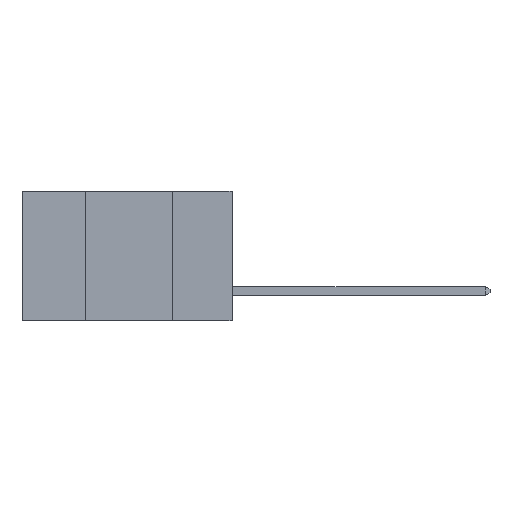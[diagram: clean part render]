
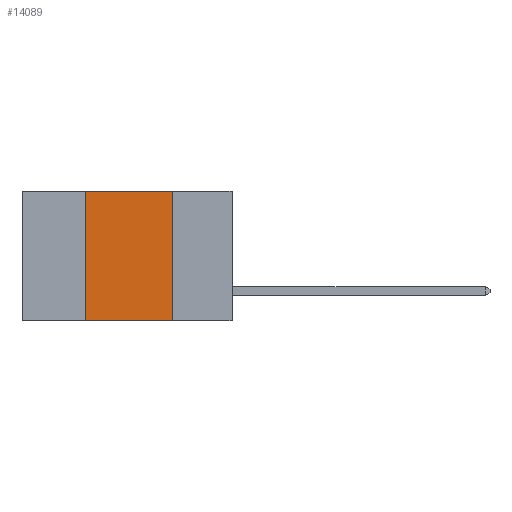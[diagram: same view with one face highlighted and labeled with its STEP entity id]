
A CAD part, left-side view. The second image highlights one B-rep face of the part: STEP entity #14089.
In plain terms, the highlighted planar face has unit normal (-1, 0, 0).
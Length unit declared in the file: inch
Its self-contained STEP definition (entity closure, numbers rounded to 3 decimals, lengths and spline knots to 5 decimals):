
#72 = EDGE_LOOP ( 'NONE', ( #18517, #10150, #10084, #10769 ) ) ;
#1150 = EDGE_CURVE ( 'NONE', #11482, #13992, #9369, .T. ) ;
#1518 = VECTOR ( 'NONE', #13849, 39.37008 ) ;
#2031 = LINE ( 'NONE', #8799, #1518 ) ;
#2563 = AXIS2_PLACEMENT_3D ( 'NONE', #2743, #13719, #4466 ) ;
#2743 = CARTESIAN_POINT ( 'NONE',  ( 0., 0.6, 0. ) ) ;
#3297 = LINE ( 'NONE', #7879, #18875 ) ;
#3384 = EDGE_CURVE ( 'NONE', #13992, #12491, #2031, .T. ) ;
#4466 = DIRECTION ( 'NONE',  ( 0., 0., -1. ) ) ;
#4492 = EDGE_CURVE ( 'NONE', #11482, #5430, #3297, .T. ) ;
#5430 = VERTEX_POINT ( 'NONE', #15774 ) ;
#6145 = VECTOR ( 'NONE', #15938, 39.37008 ) ;
#6451 = LINE ( 'NONE', #11126, #14081 ) ;
#6978 = FACE_OUTER_BOUND ( 'NONE', #72, .T. ) ;
#7617 = PLANE ( 'NONE',  #2563 ) ;
#7879 = CARTESIAN_POINT ( 'NONE',  ( 0., 0.6, -0.37 ) ) ;
#8799 = CARTESIAN_POINT ( 'NONE',  ( 0., 0.6, 0. ) ) ;
#9068 = DIRECTION ( 'NONE',  ( 0., -1., 0. ) ) ;
#9369 = LINE ( 'NONE', #15669, #6145 ) ;
#9662 = DIRECTION ( 'NONE',  ( 0., 0., -1. ) ) ;
#10084 = ORIENTED_EDGE ( 'NONE', *, *, #1150, .F. ) ;
#10150 = ORIENTED_EDGE ( 'NONE', *, *, #3384, .F. ) ;
#10769 = ORIENTED_EDGE ( 'NONE', *, *, #4492, .T. ) ;
#11126 = CARTESIAN_POINT ( 'NONE',  ( 0., 0.17, 0. ) ) ;
#11482 = VERTEX_POINT ( 'NONE', #14556 ) ;
#12491 = VERTEX_POINT ( 'NONE', #18179 ) ;
#13467 = CARTESIAN_POINT ( 'NONE',  ( 0., 0.42, 0. ) ) ;
#13719 = DIRECTION ( 'NONE',  ( 1., 0., 0. ) ) ;
#13849 = DIRECTION ( 'NONE',  ( 0., -1., 0. ) ) ;
#13992 = VERTEX_POINT ( 'NONE', #13467 ) ;
#14081 = VECTOR ( 'NONE', #9662, 39.37008 ) ;
#14089 = ADVANCED_FACE ( 'NONE', ( #6978 ), #7617, .F. ) ;
#14556 = CARTESIAN_POINT ( 'NONE',  ( 0., 0.42, -0.37 ) ) ;
#15669 = CARTESIAN_POINT ( 'NONE',  ( 0., 0.42, 0. ) ) ;
#15774 = CARTESIAN_POINT ( 'NONE',  ( 0., 0.17, -0.37 ) ) ;
#15938 = DIRECTION ( 'NONE',  ( 0., 0., 1. ) ) ;
#16739 = EDGE_CURVE ( 'NONE', #12491, #5430, #6451, .T. ) ;
#18179 = CARTESIAN_POINT ( 'NONE',  ( 0., 0.17, 0. ) ) ;
#18517 = ORIENTED_EDGE ( 'NONE', *, *, #16739, .F. ) ;
#18875 = VECTOR ( 'NONE', #9068, 39.37008 ) ;
